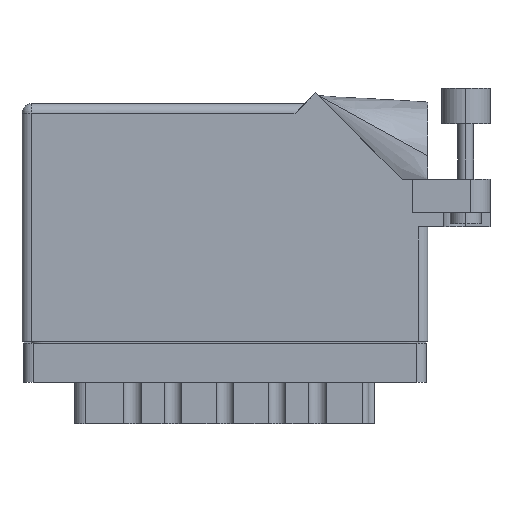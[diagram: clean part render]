
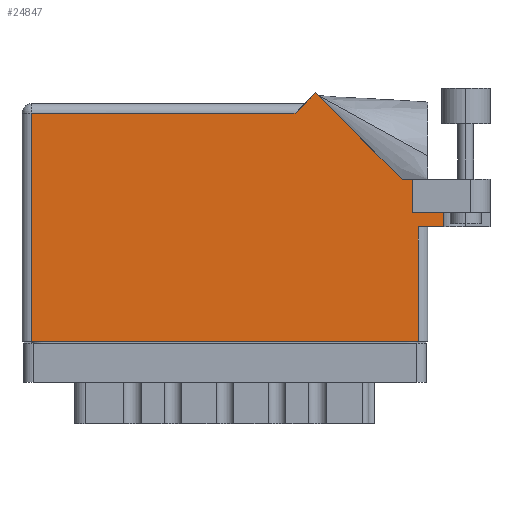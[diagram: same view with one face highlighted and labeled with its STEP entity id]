
A CAD part, front view. The second image highlights one B-rep face of the part: STEP entity #24847.
In plain terms, the highlighted face is planar.
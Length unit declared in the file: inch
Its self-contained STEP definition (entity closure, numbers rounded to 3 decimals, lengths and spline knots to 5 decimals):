
#348 = FACE_OUTER_BOUND ( 'NONE', #20838, .T. ) ;
#692 = VERTEX_POINT ( 'NONE', #32659 ) ;
#1086 = CARTESIAN_POINT ( 'NONE',  ( 0.062, 1.468, 0. ) ) ;
#2082 = VERTEX_POINT ( 'NONE', #34713 ) ;
#2276 = ORIENTED_EDGE ( 'NONE', *, *, #8267, .T. ) ;
#2318 = ORIENTED_EDGE ( 'NONE', *, *, #22016, .T. ) ;
#2553 = CARTESIAN_POINT ( 'NONE',  ( 2.44642, 1.044, 0. ) ) ;
#2628 = ORIENTED_EDGE ( 'NONE', *, *, #6507, .T. ) ;
#2783 = PLANE ( 'NONE',  #9023 ) ;
#2897 = EDGE_CURVE ( 'NONE', #19597, #27910, #28485, .T. ) ;
#2929 = DIRECTION ( 'NONE',  ( 1., 0., 0. ) ) ;
#3871 = ORIENTED_EDGE ( 'NONE', *, *, #37610, .F. ) ;
#4099 = VERTEX_POINT ( 'NONE', #13992 ) ;
#4401 = LINE ( 'NONE', #41190, #34353 ) ;
#4965 = VECTOR ( 'NONE', #36480, 39.37008 ) ;
#5192 = EDGE_CURVE ( 'NONE', #48396, #34078, #51372, .T. ) ;
#5197 = CARTESIAN_POINT ( 'NONE',  ( 1.819, 1.53, 0. ) ) ;
#5488 = VECTOR ( 'NONE', #36738, 39.37008 ) ;
#5754 = ORIENTED_EDGE ( 'NONE', *, *, #52512, .T. ) ;
#5934 = ORIENTED_EDGE ( 'NONE', *, *, #5192, .T. ) ;
#6085 = LINE ( 'NONE', #13691, #22405 ) ;
#6507 = EDGE_CURVE ( 'NONE', #47537, #38299, #4401, .T. ) ;
#6609 = CARTESIAN_POINT ( 'NONE',  ( 2.7135, 0.831, 0. ) ) ;
#6913 = CARTESIAN_POINT ( 'NONE',  ( 2.55, 0., 0. ) ) ;
#8101 = EDGE_CURVE ( 'NONE', #692, #48396, #40073, .T. ) ;
#8267 = EDGE_CURVE ( 'NONE', #43059, #4099, #45205, .T. ) ;
#9023 = AXIS2_PLACEMENT_3D ( 'NONE', #44408, #44059, #23696 ) ;
#9409 = DIRECTION ( 'NONE',  ( -0.707, -0.707, 0. ) ) ;
#9461 = CARTESIAN_POINT ( 'NONE',  ( 2.512, 0.831, 0. ) ) ;
#9755 = CARTESIAN_POINT ( 'NONE',  ( 1.88971, 1.60071, 0. ) ) ;
#11084 = ORIENTED_EDGE ( 'NONE', *, *, #17523, .T. ) ;
#12224 = VECTOR ( 'NONE', #13644, 39.37008 ) ;
#12628 = CARTESIAN_POINT ( 'NONE',  ( 1.757, 1.468, 0. ) ) ;
#13644 = DIRECTION ( 'NONE',  ( 1., 0., 0. ) ) ;
#13656 = VERTEX_POINT ( 'NONE', #44834 ) ;
#13691 = CARTESIAN_POINT ( 'NONE',  ( 2.7135, 1.16177, 0. ) ) ;
#13992 = CARTESIAN_POINT ( 'NONE',  ( 0.062, 0., 0. ) ) ;
#14719 = CARTESIAN_POINT ( 'NONE',  ( 2.55, 0.737, 0. ) ) ;
#14834 = CARTESIAN_POINT ( 'NONE',  ( 3.012, 1.044, 0. ) ) ;
#16142 = LINE ( 'NONE', #19893, #26520 ) ;
#16825 = ORIENTED_EDGE ( 'NONE', *, *, #2897, .F. ) ;
#17523 = EDGE_CURVE ( 'NONE', #13656, #692, #45079, .T. ) ;
#18181 = VECTOR ( 'NONE', #9409, 39.37008 ) ;
#19227 = CARTESIAN_POINT ( 'NONE',  ( 0., 0., 0. ) ) ;
#19597 = VERTEX_POINT ( 'NONE', #21567 ) ;
#19714 = DIRECTION ( 'NONE',  ( 0., 1., 0. ) ) ;
#19740 = DIRECTION ( 'NONE',  ( -1., 0., 0. ) ) ;
#19893 = CARTESIAN_POINT ( 'NONE',  ( 2.512, 0.831, 0. ) ) ;
#19976 = ORIENTED_EDGE ( 'NONE', *, *, #8101, .T. ) ;
#20464 = DIRECTION ( 'NONE',  ( 0., 1., 0. ) ) ;
#20838 = EDGE_LOOP ( 'NONE', ( #27105, #2628, #2318, #3871, #16825, #5754, #11084, #19976, #5934, #52751, #2276 ) ) ;
#21567 = CARTESIAN_POINT ( 'NONE',  ( 2.512, 0.831, 0. ) ) ;
#22016 = EDGE_CURVE ( 'NONE', #38299, #2082, #31683, .T. ) ;
#22070 = DIRECTION ( 'NONE',  ( 0., -1., 0. ) ) ;
#22405 = VECTOR ( 'NONE', #22070, 39.37008 ) ;
#23285 = DIRECTION ( 'NONE',  ( -0.707, 0.707, 0. ) ) ;
#23696 = DIRECTION ( 'NONE',  ( -1., 0., 0. ) ) ;
#24847 = ADVANCED_FACE ( 'NONE', ( #348 ), #2783, .F. ) ;
#26520 = VECTOR ( 'NONE', #19714, 39.37008 ) ;
#27105 = ORIENTED_EDGE ( 'NONE', *, *, #53711, .T. ) ;
#27910 = VERTEX_POINT ( 'NONE', #6609 ) ;
#28485 = LINE ( 'NONE', #9461, #12224 ) ;
#28988 = VECTOR ( 'NONE', #23285, 39.37008 ) ;
#30374 = VECTOR ( 'NONE', #2929, 39.37008 ) ;
#31683 = LINE ( 'NONE', #34959, #30374 ) ;
#31808 = CARTESIAN_POINT ( 'NONE',  ( 0., 1.468, 0. ) ) ;
#32535 = CARTESIAN_POINT ( 'NONE',  ( 0.062, 0., 0. ) ) ;
#32659 = CARTESIAN_POINT ( 'NONE',  ( 2.44642, 1.044, 0. ) ) ;
#34078 = VERTEX_POINT ( 'NONE', #12628 ) ;
#34353 = VECTOR ( 'NONE', #20464, 39.37008 ) ;
#34713 = CARTESIAN_POINT ( 'NONE',  ( 2.7135, 0.737, 0. ) ) ;
#34959 = CARTESIAN_POINT ( 'NONE',  ( 2.612, 0.737, 0. ) ) ;
#36002 = DIRECTION ( 'NONE',  ( -1., 0., 0. ) ) ;
#36480 = DIRECTION ( 'NONE',  ( 1., 0., 0. ) ) ;
#36738 = DIRECTION ( 'NONE',  ( 0., -1., 0. ) ) ;
#37610 = EDGE_CURVE ( 'NONE', #27910, #2082, #6085, .T. ) ;
#38299 = VERTEX_POINT ( 'NONE', #14719 ) ;
#40073 = LINE ( 'NONE', #2553, #28988 ) ;
#40468 = VECTOR ( 'NONE', #36002, 39.37008 ) ;
#41190 = CARTESIAN_POINT ( 'NONE',  ( 2.55, 0.737, 0. ) ) ;
#43059 = VERTEX_POINT ( 'NONE', #1086 ) ;
#44059 = DIRECTION ( 'NONE',  ( 0., 0., -1. ) ) ;
#44408 = CARTESIAN_POINT ( 'NONE',  ( 0., 1.53, 0. ) ) ;
#44641 = EDGE_CURVE ( 'NONE', #34078, #43059, #48313, .T. ) ;
#44834 = CARTESIAN_POINT ( 'NONE',  ( 2.512, 1.044, 0. ) ) ;
#45079 = LINE ( 'NONE', #14834, #52250 ) ;
#45205 = LINE ( 'NONE', #32535, #5488 ) ;
#45300 = LINE ( 'NONE', #19227, #4965 ) ;
#47537 = VERTEX_POINT ( 'NONE', #6913 ) ;
#48313 = LINE ( 'NONE', #31808, #40468 ) ;
#48396 = VERTEX_POINT ( 'NONE', #9755 ) ;
#51372 = LINE ( 'NONE', #5197, #18181 ) ;
#52250 = VECTOR ( 'NONE', #19740, 39.37008 ) ;
#52512 = EDGE_CURVE ( 'NONE', #19597, #13656, #16142, .T. ) ;
#52751 = ORIENTED_EDGE ( 'NONE', *, *, #44641, .T. ) ;
#53711 = EDGE_CURVE ( 'NONE', #4099, #47537, #45300, .T. ) ;
